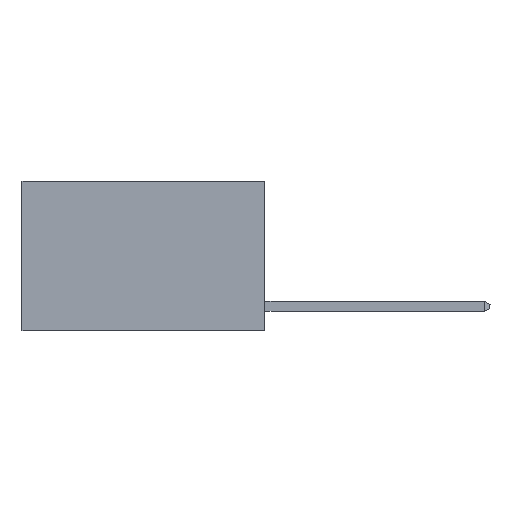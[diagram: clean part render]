
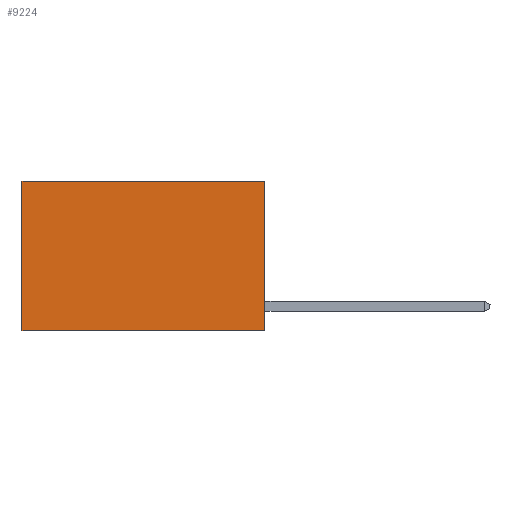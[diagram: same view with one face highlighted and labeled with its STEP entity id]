
A CAD part, left-side view. The second image highlights one B-rep face of the part: STEP entity #9224.
In plain terms, the highlighted planar face has unit normal (-1, 0, 0).
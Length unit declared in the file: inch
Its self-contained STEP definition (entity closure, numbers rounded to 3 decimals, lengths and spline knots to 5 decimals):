
#100 = LINE ( 'NONE', #9553, #1971 ) ;
#631 = EDGE_CURVE ( 'NONE', #1450, #2106, #100, .T. ) ;
#778 = DIRECTION ( 'NONE',  ( 0., 1., 0. ) ) ;
#857 = VECTOR ( 'NONE', #7364, 39.37008 ) ;
#1450 = VERTEX_POINT ( 'NONE', #10962 ) ;
#1558 = DIRECTION ( 'NONE',  ( 1., 0., 0. ) ) ;
#1971 = VECTOR ( 'NONE', #3452, 39.37008 ) ;
#2106 = VERTEX_POINT ( 'NONE', #11288 ) ;
#3452 = DIRECTION ( 'NONE',  ( 0., 0., -1. ) ) ;
#5069 = EDGE_CURVE ( 'NONE', #22977, #1450, #19228, .T. ) ;
#7364 = DIRECTION ( 'NONE',  ( 0., 0., -1. ) ) ;
#8200 = CARTESIAN_POINT ( 'NONE',  ( 0.2625, 0., 0. ) ) ;
#8308 = CARTESIAN_POINT ( 'NONE',  ( 0.2625, 0., -0.37 ) ) ;
#9142 = ORIENTED_EDGE ( 'NONE', *, *, #5069, .T. ) ;
#9224 = ADVANCED_FACE ( 'NONE', ( #21543 ), #11239, .F. ) ;
#9553 = CARTESIAN_POINT ( 'NONE',  ( 0.2625, 0.6, 0. ) ) ;
#10211 = LINE ( 'NONE', #15487, #857 ) ;
#10527 = VECTOR ( 'NONE', #778, 39.37008 ) ;
#10962 = CARTESIAN_POINT ( 'NONE',  ( 0.2625, 0.6, 0. ) ) ;
#11239 = PLANE ( 'NONE',  #14266 ) ;
#11288 = CARTESIAN_POINT ( 'NONE',  ( 0.2625, 0.6, -0.37 ) ) ;
#11688 = VECTOR ( 'NONE', #12674, 39.37008 ) ;
#12674 = DIRECTION ( 'NONE',  ( 0., 1., 0. ) ) ;
#13314 = ORIENTED_EDGE ( 'NONE', *, *, #631, .T. ) ;
#13969 = ORIENTED_EDGE ( 'NONE', *, *, #24927, .F. ) ;
#14266 = AXIS2_PLACEMENT_3D ( 'NONE', #25199, #1558, #17364 ) ;
#15487 = CARTESIAN_POINT ( 'NONE',  ( 0.2625, 0., 0. ) ) ;
#15820 = VERTEX_POINT ( 'NONE', #8308 ) ;
#15850 = LINE ( 'NONE', #19045, #10527 ) ;
#17364 = DIRECTION ( 'NONE',  ( 0., 0., -1. ) ) ;
#19045 = CARTESIAN_POINT ( 'NONE',  ( 0.2625, 0., -0.37 ) ) ;
#19228 = LINE ( 'NONE', #24999, #11688 ) ;
#19918 = EDGE_LOOP ( 'NONE', ( #13314, #13969, #24189, #9142 ) ) ;
#21543 = FACE_OUTER_BOUND ( 'NONE', #19918, .T. ) ;
#22977 = VERTEX_POINT ( 'NONE', #8200 ) ;
#24189 = ORIENTED_EDGE ( 'NONE', *, *, #25145, .F. ) ;
#24927 = EDGE_CURVE ( 'NONE', #15820, #2106, #15850, .T. ) ;
#24999 = CARTESIAN_POINT ( 'NONE',  ( 0.2625, 0., 0. ) ) ;
#25145 = EDGE_CURVE ( 'NONE', #22977, #15820, #10211, .T. ) ;
#25199 = CARTESIAN_POINT ( 'NONE',  ( 0.2625, 0., 0. ) ) ;
